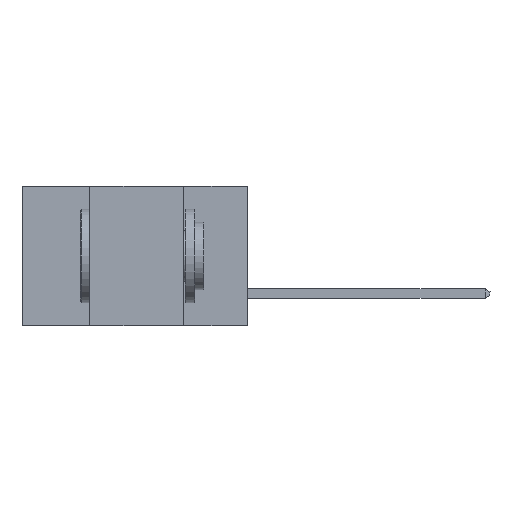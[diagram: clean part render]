
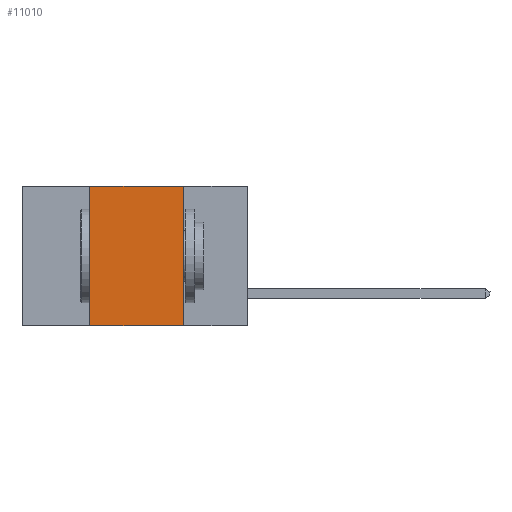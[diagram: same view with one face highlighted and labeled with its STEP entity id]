
A CAD part, left-side view. The second image highlights one B-rep face of the part: STEP entity #11010.
In plain terms, the highlighted planar face has unit normal (-1, 0, 0).
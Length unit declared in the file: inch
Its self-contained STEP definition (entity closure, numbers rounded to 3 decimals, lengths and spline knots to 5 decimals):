
#72 = CARTESIAN_POINT ( 'NONE',  ( 0., 0.17, -0.37 ) ) ;
#158 = LINE ( 'NONE', #10361, #1661 ) ;
#497 = CARTESIAN_POINT ( 'NONE',  ( 0., 0.6, 0. ) ) ;
#612 = CARTESIAN_POINT ( 'NONE',  ( 0., 0.17, -0.37 ) ) ;
#1560 = AXIS2_PLACEMENT_3D ( 'NONE', #6955, #7062, #5392 ) ;
#1574 = CARTESIAN_POINT ( 'NONE',  ( 0., 0.42, 0. ) ) ;
#1661 = VECTOR ( 'NONE', #3593, 39.37008 ) ;
#1904 = VERTEX_POINT ( 'NONE', #2723 ) ;
#2223 = DIRECTION ( 'NONE',  ( 0., -1., 0. ) ) ;
#2723 = CARTESIAN_POINT ( 'NONE',  ( 0., 0.17, 0. ) ) ;
#3044 = ORIENTED_EDGE ( 'NONE', *, *, #4579, .F. ) ;
#3245 = VERTEX_POINT ( 'NONE', #10397 ) ;
#3353 = CARTESIAN_POINT ( 'NONE',  ( 0., 0.6, -0.37 ) ) ;
#3593 = DIRECTION ( 'NONE',  ( 0., 0., 1. ) ) ;
#4579 = EDGE_CURVE ( 'NONE', #3245, #7315, #158, .T. ) ;
#4581 = VECTOR ( 'NONE', #10068, 39.37008 ) ;
#4976 = VECTOR ( 'NONE', #6571, 39.37008 ) ;
#5140 = LINE ( 'NONE', #3353, #4581 ) ;
#5367 = VERTEX_POINT ( 'NONE', #72 ) ;
#5392 = DIRECTION ( 'NONE',  ( 0., 0., -1. ) ) ;
#6165 = FACE_OUTER_BOUND ( 'NONE', #6976, .T. ) ;
#6571 = DIRECTION ( 'NONE',  ( 0., 0., -1. ) ) ;
#6955 = CARTESIAN_POINT ( 'NONE',  ( 0., 0.6, 0. ) ) ;
#6976 = EDGE_LOOP ( 'NONE', ( #9559, #9410, #3044, #7088 ) ) ;
#7062 = DIRECTION ( 'NONE',  ( 1., 0., 0. ) ) ;
#7088 = ORIENTED_EDGE ( 'NONE', *, *, #9492, .T. ) ;
#7315 = VERTEX_POINT ( 'NONE', #1574 ) ;
#7345 = LINE ( 'NONE', #497, #7965 ) ;
#7965 = VECTOR ( 'NONE', #2223, 39.37008 ) ;
#9410 = ORIENTED_EDGE ( 'NONE', *, *, #9427, .F. ) ;
#9427 = EDGE_CURVE ( 'NONE', #7315, #1904, #7345, .T. ) ;
#9463 = PLANE ( 'NONE',  #1560 ) ;
#9492 = EDGE_CURVE ( 'NONE', #3245, #5367, #5140, .T. ) ;
#9559 = ORIENTED_EDGE ( 'NONE', *, *, #10737, .F. ) ;
#10068 = DIRECTION ( 'NONE',  ( 0., -1., 0. ) ) ;
#10361 = CARTESIAN_POINT ( 'NONE',  ( 0., 0.42, -0.37 ) ) ;
#10397 = CARTESIAN_POINT ( 'NONE',  ( 0., 0.42, -0.37 ) ) ;
#10737 = EDGE_CURVE ( 'NONE', #1904, #5367, #10859, .T. ) ;
#10859 = LINE ( 'NONE', #612, #4976 ) ;
#11010 = ADVANCED_FACE ( 'NONE', ( #6165 ), #9463, .F. ) ;
